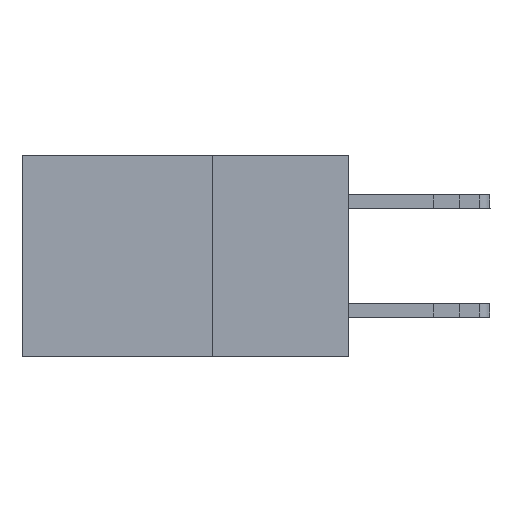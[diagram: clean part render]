
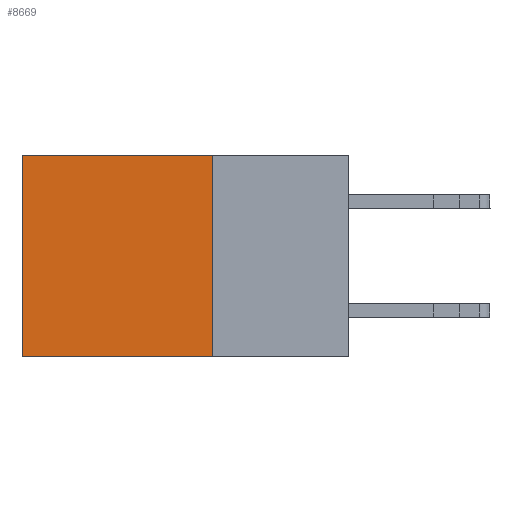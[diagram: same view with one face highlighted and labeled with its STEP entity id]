
A CAD part, left-side view. The second image highlights one B-rep face of the part: STEP entity #8669.
In plain terms, the highlighted planar face has unit normal (-1, 0, 0).
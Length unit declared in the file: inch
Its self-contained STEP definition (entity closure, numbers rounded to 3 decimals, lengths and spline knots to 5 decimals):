
#125 = LINE ( 'NONE', #2233, #2321 ) ;
#175 = EDGE_CURVE ( 'NONE', #11681, #5641, #7196, .T. ) ;
#314 = LINE ( 'NONE', #5610, #8353 ) ;
#317 = EDGE_CURVE ( 'NONE', #5641, #1398, #314, .T. ) ;
#523 = DIRECTION ( 'NONE',  ( 0., 1., 0. ) ) ;
#719 = ORIENTED_EDGE ( 'NONE', *, *, #7084, .F. ) ;
#1398 = VERTEX_POINT ( 'NONE', #12321 ) ;
#1718 = FACE_OUTER_BOUND ( 'NONE', #2317, .T. ) ;
#2175 = DIRECTION ( 'NONE',  ( 0., 1., 0. ) ) ;
#2233 = CARTESIAN_POINT ( 'NONE',  ( 0.298, 0.25, 0. ) ) ;
#2317 = EDGE_LOOP ( 'NONE', ( #6578, #719, #11061, #12219 ) ) ;
#2321 = VECTOR ( 'NONE', #8179, 39.37008 ) ;
#2523 = VERTEX_POINT ( 'NONE', #8280 ) ;
#2891 = CARTESIAN_POINT ( 'NONE',  ( 0.298, 0.25, 0. ) ) ;
#3013 = CARTESIAN_POINT ( 'NONE',  ( 0.298, 0.25, 0. ) ) ;
#3282 = DIRECTION ( 'NONE',  ( 0., 0., -1. ) ) ;
#3697 = PLANE ( 'NONE',  #10709 ) ;
#5220 = VECTOR ( 'NONE', #2175, 39.37008 ) ;
#5610 = CARTESIAN_POINT ( 'NONE',  ( 0.298, 0.6, 0. ) ) ;
#5641 = VERTEX_POINT ( 'NONE', #12326 ) ;
#6578 = ORIENTED_EDGE ( 'NONE', *, *, #317, .T. ) ;
#7084 = EDGE_CURVE ( 'NONE', #2523, #1398, #8574, .T. ) ;
#7196 = LINE ( 'NONE', #11208, #5220 ) ;
#7368 = EDGE_CURVE ( 'NONE', #11681, #2523, #125, .T. ) ;
#7985 = DIRECTION ( 'NONE',  ( 1., 0., 0. ) ) ;
#8179 = DIRECTION ( 'NONE',  ( 0., 0., -1. ) ) ;
#8280 = CARTESIAN_POINT ( 'NONE',  ( 0.298, 0.25, -0.37 ) ) ;
#8353 = VECTOR ( 'NONE', #3282, 39.37008 ) ;
#8574 = LINE ( 'NONE', #12665, #9054 ) ;
#8669 = ADVANCED_FACE ( 'NONE', ( #1718 ), #3697, .F. ) ;
#9054 = VECTOR ( 'NONE', #523, 39.37008 ) ;
#10709 = AXIS2_PLACEMENT_3D ( 'NONE', #2891, #7985, #11738 ) ;
#11061 = ORIENTED_EDGE ( 'NONE', *, *, #7368, .F. ) ;
#11208 = CARTESIAN_POINT ( 'NONE',  ( 0.298, 0.25, 0. ) ) ;
#11681 = VERTEX_POINT ( 'NONE', #3013 ) ;
#11738 = DIRECTION ( 'NONE',  ( 0., 0., -1. ) ) ;
#12219 = ORIENTED_EDGE ( 'NONE', *, *, #175, .T. ) ;
#12321 = CARTESIAN_POINT ( 'NONE',  ( 0.298, 0.6, -0.37 ) ) ;
#12326 = CARTESIAN_POINT ( 'NONE',  ( 0.298, 0.6, 0. ) ) ;
#12665 = CARTESIAN_POINT ( 'NONE',  ( 0.298, 0.25, -0.37 ) ) ;
